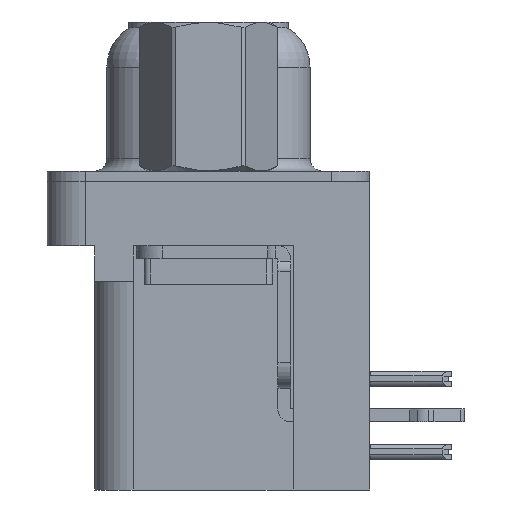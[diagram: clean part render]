
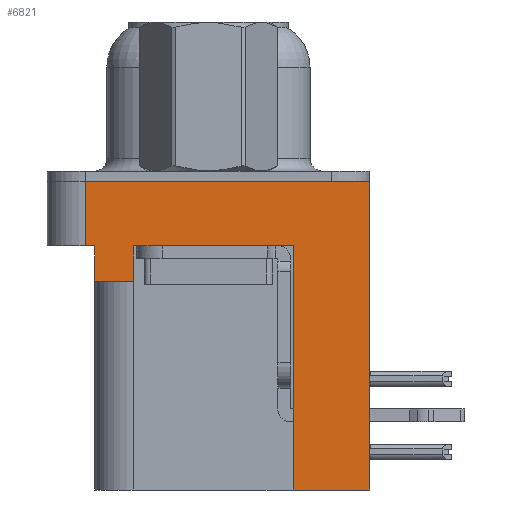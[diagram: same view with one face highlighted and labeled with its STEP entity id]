
A CAD part, left-side view. The second image highlights one B-rep face of the part: STEP entity #6821.
In plain terms, the highlighted planar face has unit normal (-1, 0, 0).
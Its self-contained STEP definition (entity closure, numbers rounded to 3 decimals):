
#66 = DIRECTION ( 'NONE',  ( 0., 0., 1. ) ) ;
#758 = LINE ( 'NONE', #17069, #25457 ) ;
#795 = VERTEX_POINT ( 'NONE', #15174 ) ;
#821 = LINE ( 'NONE', #22428, #12938 ) ;
#1406 = EDGE_CURVE ( 'NONE', #18948, #3051, #11006, .T. ) ;
#2011 = ORIENTED_EDGE ( 'NONE', *, *, #21517, .F. ) ;
#2563 = ORIENTED_EDGE ( 'NONE', *, *, #1406, .F. ) ;
#2618 = DIRECTION ( 'NONE',  ( 0., 1., 0. ) ) ;
#2773 = CARTESIAN_POINT ( 'NONE',  ( -2.935, 4.425, -2.5 ) ) ;
#2971 = DIRECTION ( 'NONE',  ( 0., 0., 1. ) ) ;
#3051 = VERTEX_POINT ( 'NONE', #26993 ) ;
#3605 = CARTESIAN_POINT ( 'NONE',  ( -2.935, -6.275, 0. ) ) ;
#3719 = ORIENTED_EDGE ( 'NONE', *, *, #23760, .F. ) ;
#3822 = LINE ( 'NONE', #18475, #28887 ) ;
#3853 = ORIENTED_EDGE ( 'NONE', *, *, #9650, .F. ) ;
#4115 = VECTOR ( 'NONE', #4252, 1000. ) ;
#4252 = DIRECTION ( 'NONE',  ( 0., 1., 0. ) ) ;
#4343 = VECTOR ( 'NONE', #2618, 1000. ) ;
#4516 = EDGE_CURVE ( 'NONE', #795, #3051, #22934, .T. ) ;
#4758 = VERTEX_POINT ( 'NONE', #30413 ) ;
#5117 = LINE ( 'NONE', #22143, #4343 ) ;
#5155 = CARTESIAN_POINT ( 'NONE',  ( -2.935, -6.275, -2.5 ) ) ;
#5565 = EDGE_CURVE ( 'NONE', #27503, #795, #821, .T. ) ;
#6821 = ADVANCED_FACE ( 'NONE', ( #29654 ), #15340, .T. ) ;
#7386 = EDGE_LOOP ( 'NONE', ( #17456, #2011, #12022, #3719, #7764, #29424, #23283, #2563, #3853, #30933 ) ) ;
#7719 = VECTOR ( 'NONE', #9186, 1000. ) ;
#7764 = ORIENTED_EDGE ( 'NONE', *, *, #23602, .F. ) ;
#8249 = DIRECTION ( 'NONE',  ( -1., 0., 0. ) ) ;
#8909 = CARTESIAN_POINT ( 'NONE',  ( -2.935, -6.275, -12. ) ) ;
#9186 = DIRECTION ( 'NONE',  ( 0., -1., 0. ) ) ;
#9650 = EDGE_CURVE ( 'NONE', #26980, #18948, #24568, .T. ) ;
#10002 = LINE ( 'NONE', #3605, #7719 ) ;
#10789 = VECTOR ( 'NONE', #17245, 1000. ) ;
#11006 = LINE ( 'NONE', #13446, #28880 ) ;
#11175 = DIRECTION ( 'NONE',  ( 0., -1., 0. ) ) ;
#12022 = ORIENTED_EDGE ( 'NONE', *, *, #30504, .T. ) ;
#12037 = AXIS2_PLACEMENT_3D ( 'NONE', #19938, #8249, #2971 ) ;
#12938 = VECTOR ( 'NONE', #14876, 1000. ) ;
#13299 = CARTESIAN_POINT ( 'NONE',  ( -2.935, 4.775, 0. ) ) ;
#13446 = CARTESIAN_POINT ( 'NONE',  ( -2.935, -3.295, -12. ) ) ;
#14865 = VERTEX_POINT ( 'NONE', #29682 ) ;
#14876 = DIRECTION ( 'NONE',  ( 0., 0., 1. ) ) ;
#15174 = CARTESIAN_POINT ( 'NONE',  ( -2.935, 2.895, -2.5 ) ) ;
#15340 = PLANE ( 'NONE',  #12037 ) ;
#15611 = LINE ( 'NONE', #23368, #17523 ) ;
#16129 = DIRECTION ( 'NONE',  ( 0., 0., 1. ) ) ;
#17069 = CARTESIAN_POINT ( 'NONE',  ( -2.935, -6.275, -2.5 ) ) ;
#17245 = DIRECTION ( 'NONE',  ( 0., -1., 0. ) ) ;
#17368 = CARTESIAN_POINT ( 'NONE',  ( -2.935, 4.775, -2.5 ) ) ;
#17456 = ORIENTED_EDGE ( 'NONE', *, *, #20234, .F. ) ;
#17523 = VECTOR ( 'NONE', #11175, 1000. ) ;
#17786 = DIRECTION ( 'NONE',  ( 0., 0., 1. ) ) ;
#18475 = CARTESIAN_POINT ( 'NONE',  ( -2.935, 4.425, -3.9 ) ) ;
#18747 = CARTESIAN_POINT ( 'NONE',  ( -2.935, -3.295, -12. ) ) ;
#18948 = VERTEX_POINT ( 'NONE', #22485 ) ;
#19938 = CARTESIAN_POINT ( 'NONE',  ( -2.935, -6.275, -2.5 ) ) ;
#20234 = EDGE_CURVE ( 'NONE', #24682, #14865, #10002, .T. ) ;
#21517 = EDGE_CURVE ( 'NONE', #30496, #24682, #27412, .T. ) ;
#22143 = CARTESIAN_POINT ( 'NONE',  ( -2.935, 4.425, -3.9 ) ) ;
#22428 = CARTESIAN_POINT ( 'NONE',  ( -2.935, 2.895, -3.9 ) ) ;
#22473 = EDGE_CURVE ( 'NONE', #26980, #14865, #758, .T. ) ;
#22485 = CARTESIAN_POINT ( 'NONE',  ( -2.935, -3.295, -12. ) ) ;
#22934 = LINE ( 'NONE', #5155, #10789 ) ;
#23283 = ORIENTED_EDGE ( 'NONE', *, *, #4516, .T. ) ;
#23306 = CARTESIAN_POINT ( 'NONE',  ( -2.935, 2.895, -3.9 ) ) ;
#23368 = CARTESIAN_POINT ( 'NONE',  ( -2.935, -6.275, -2.5 ) ) ;
#23602 = EDGE_CURVE ( 'NONE', #27503, #4758, #5117, .T. ) ;
#23760 = EDGE_CURVE ( 'NONE', #4758, #31341, #3822, .T. ) ;
#24568 = LINE ( 'NONE', #18747, #4115 ) ;
#24682 = VERTEX_POINT ( 'NONE', #13299 ) ;
#25457 = VECTOR ( 'NONE', #17786, 1000. ) ;
#25712 = CARTESIAN_POINT ( 'NONE',  ( -2.935, 4.775, -2.5 ) ) ;
#26980 = VERTEX_POINT ( 'NONE', #8909 ) ;
#26993 = CARTESIAN_POINT ( 'NONE',  ( -2.935, -3.295, -2.5 ) ) ;
#27412 = LINE ( 'NONE', #17368, #30889 ) ;
#27503 = VERTEX_POINT ( 'NONE', #23306 ) ;
#28880 = VECTOR ( 'NONE', #30499, 1000. ) ;
#28887 = VECTOR ( 'NONE', #16129, 1000. ) ;
#29424 = ORIENTED_EDGE ( 'NONE', *, *, #5565, .T. ) ;
#29654 = FACE_OUTER_BOUND ( 'NONE', #7386, .T. ) ;
#29682 = CARTESIAN_POINT ( 'NONE',  ( -2.935, -6.275, 0. ) ) ;
#30413 = CARTESIAN_POINT ( 'NONE',  ( -2.935, 4.425, -3.9 ) ) ;
#30496 = VERTEX_POINT ( 'NONE', #25712 ) ;
#30499 = DIRECTION ( 'NONE',  ( 0., 0., 1. ) ) ;
#30504 = EDGE_CURVE ( 'NONE', #30496, #31341, #15611, .T. ) ;
#30889 = VECTOR ( 'NONE', #66, 1000. ) ;
#30933 = ORIENTED_EDGE ( 'NONE', *, *, #22473, .T. ) ;
#31341 = VERTEX_POINT ( 'NONE', #2773 ) ;
